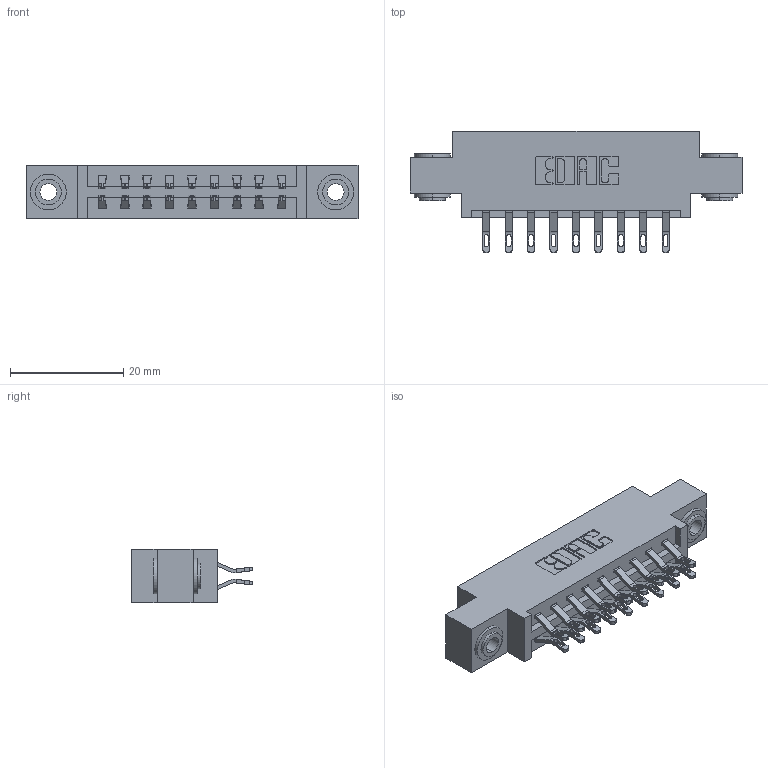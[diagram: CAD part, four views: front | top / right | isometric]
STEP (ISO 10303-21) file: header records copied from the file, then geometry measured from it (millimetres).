
FILE_DESCRIPTION (( 'STEP AP203' ), '1' );
FILE_NAME ('387-018-555-803.STEP', '2019-10-16T01:45:53', ( '' ), ( '' ), 'SwSTEP 2.0', 'SolidWorks 2016', '' );
FILE_SCHEMA (( 'CONFIG_CONTROL_DESIGN' ));
Length unit declared in the file: inch
Products named in the file (4): 387-018-555-803; 337 Part_0.170 Offset - 0.156 Dia-TH; 345-292-001_555 Tail; 345-250-002_345-250-002-102
Assembly tree (21 placements, depth 2):
  387-018-555-803
    337 Part_0.170 Offset - 0.156 Dia-TH
    345-292-001_555 Tail  x18
    345-250-002_345-250-002-102  x2
Bounding box: 58.67 x 21.47 x 9.4 mm (x, y, z)
Volume: 5698.4 mm3; surface area: 6650.5 mm2
Topology: 21 solids, 21 shells, 1236 faces, 3801 edges, 2530 vertices
Faces by surface type: plane 732, cylinder 496, cone 8
Entity records: 12354 total; most frequent: CARTESIAN_POINT 2119, ORIENTED_EDGE 2018, DIRECTION 1867, EDGE_CURVE 1009, VECTOR 837, LINE 837, VERTEX_POINT 670, AXIS2_PLACEMENT_3D 515
